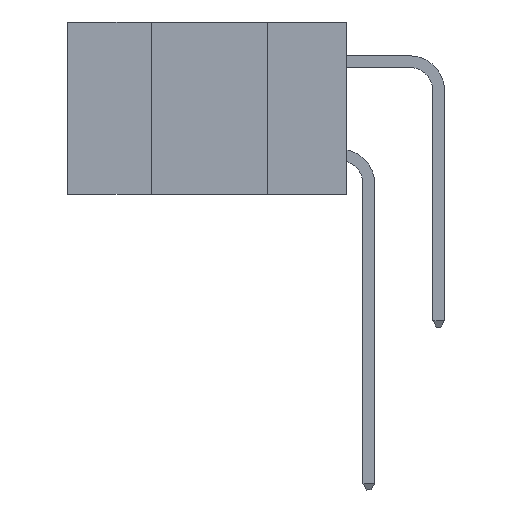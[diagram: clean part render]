
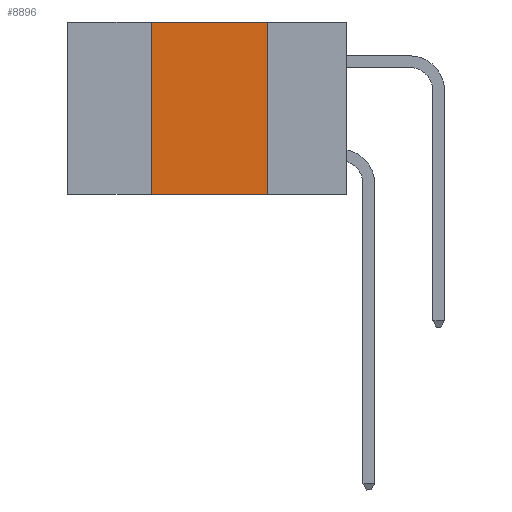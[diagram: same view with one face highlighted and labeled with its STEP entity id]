
A CAD part, left-side view. The second image highlights one B-rep face of the part: STEP entity #8896.
In plain terms, the highlighted planar face has unit normal (-1, 0, 0).
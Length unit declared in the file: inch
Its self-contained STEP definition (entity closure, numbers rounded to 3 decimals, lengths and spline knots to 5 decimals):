
#440 = EDGE_CURVE ( 'NONE', #4949, #10540, #11445, .T. ) ;
#504 = LINE ( 'NONE', #6250, #10515 ) ;
#829 = EDGE_CURVE ( 'NONE', #12548, #4949, #504, .T. ) ;
#1102 = CARTESIAN_POINT ( 'NONE',  ( 0., 0.6, 0. ) ) ;
#1322 = VERTEX_POINT ( 'NONE', #11089 ) ;
#2155 = PLANE ( 'NONE',  #12590 ) ;
#2275 = CARTESIAN_POINT ( 'NONE',  ( 0., 0.6, 0. ) ) ;
#4337 = LINE ( 'NONE', #4983, #11509 ) ;
#4618 = ORIENTED_EDGE ( 'NONE', *, *, #10356, .T. ) ;
#4652 = VECTOR ( 'NONE', #4770, 39.37008 ) ;
#4770 = DIRECTION ( 'NONE',  ( 0., -1., 0. ) ) ;
#4937 = DIRECTION ( 'NONE',  ( 0., 0., -1. ) ) ;
#4949 = VERTEX_POINT ( 'NONE', #6868 ) ;
#4983 = CARTESIAN_POINT ( 'NONE',  ( 0., 0.17, 0. ) ) ;
#5074 = CARTESIAN_POINT ( 'NONE',  ( 0., 0.17, 0. ) ) ;
#6250 = CARTESIAN_POINT ( 'NONE',  ( 0., 0.42, 0. ) ) ;
#6355 = DIRECTION ( 'NONE',  ( 0., 0., -1. ) ) ;
#6868 = CARTESIAN_POINT ( 'NONE',  ( 0., 0.42, 0. ) ) ;
#7311 = ORIENTED_EDGE ( 'NONE', *, *, #12642, .F. ) ;
#7340 = LINE ( 'NONE', #11317, #4652 ) ;
#7463 = EDGE_LOOP ( 'NONE', ( #7311, #7464, #11485, #4618 ) ) ;
#7464 = ORIENTED_EDGE ( 'NONE', *, *, #440, .F. ) ;
#7839 = FACE_OUTER_BOUND ( 'NONE', #7463, .T. ) ;
#7890 = CARTESIAN_POINT ( 'NONE',  ( 0., 0.42, -0.37 ) ) ;
#8896 = ADVANCED_FACE ( 'NONE', ( #7839 ), #2155, .F. ) ;
#9385 = DIRECTION ( 'NONE',  ( 0., -1., 0. ) ) ;
#10356 = EDGE_CURVE ( 'NONE', #12548, #1322, #7340, .T. ) ;
#10515 = VECTOR ( 'NONE', #12631, 39.37008 ) ;
#10540 = VERTEX_POINT ( 'NONE', #5074 ) ;
#11089 = CARTESIAN_POINT ( 'NONE',  ( 0., 0.17, -0.37 ) ) ;
#11163 = VECTOR ( 'NONE', #9385, 39.37008 ) ;
#11317 = CARTESIAN_POINT ( 'NONE',  ( 0., 0.6, -0.37 ) ) ;
#11445 = LINE ( 'NONE', #2275, #11163 ) ;
#11485 = ORIENTED_EDGE ( 'NONE', *, *, #829, .F. ) ;
#11509 = VECTOR ( 'NONE', #4937, 39.37008 ) ;
#11843 = DIRECTION ( 'NONE',  ( 1., 0., 0. ) ) ;
#12548 = VERTEX_POINT ( 'NONE', #7890 ) ;
#12590 = AXIS2_PLACEMENT_3D ( 'NONE', #1102, #11843, #6355 ) ;
#12631 = DIRECTION ( 'NONE',  ( 0., 0., 1. ) ) ;
#12642 = EDGE_CURVE ( 'NONE', #10540, #1322, #4337, .T. ) ;
